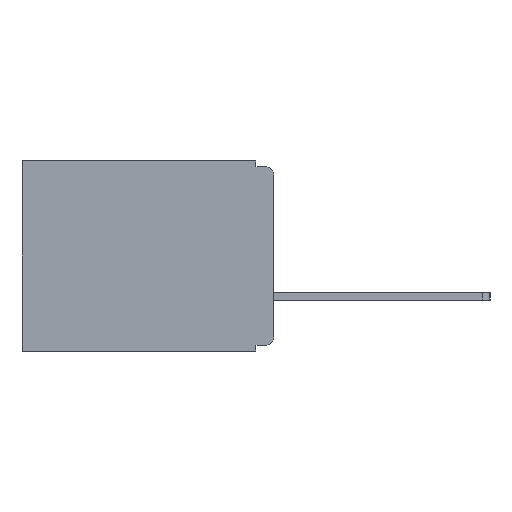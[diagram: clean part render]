
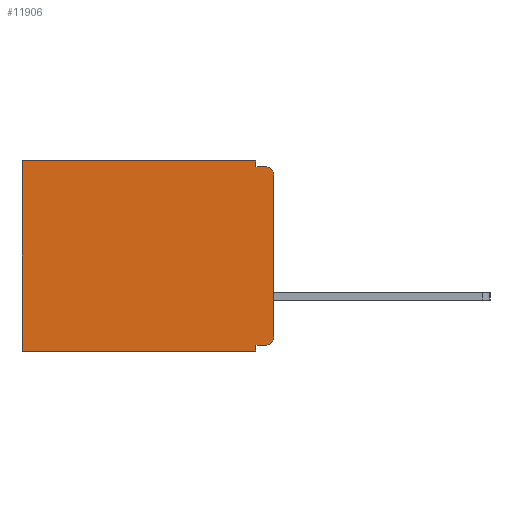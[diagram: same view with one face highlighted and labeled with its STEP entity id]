
A CAD part, left-side view. The second image highlights one B-rep face of the part: STEP entity #11906.
In plain terms, the highlighted planar face has unit normal (-1, 0, 0).
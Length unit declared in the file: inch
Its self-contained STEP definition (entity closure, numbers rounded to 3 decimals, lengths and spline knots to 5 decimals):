
#250 = AXIS2_PLACEMENT_3D ( 'NONE', #4049, #21168, #6512 ) ;
#1176 = CARTESIAN_POINT ( 'NONE',  ( 0.3, 0., -0.33 ) ) ;
#1823 = VECTOR ( 'NONE', #9104, 39.37008 ) ;
#1893 = VERTEX_POINT ( 'NONE', #15947 ) ;
#1997 = VERTEX_POINT ( 'NONE', #14978 ) ;
#2193 = EDGE_CURVE ( 'NONE', #8790, #23885, #7964, .T. ) ;
#3011 = VECTOR ( 'NONE', #12356, 39.37008 ) ;
#3123 = ORIENTED_EDGE ( 'NONE', *, *, #17317, .T. ) ;
#3446 = CARTESIAN_POINT ( 'NONE',  ( 0.3, 0.437, -0.33 ) ) ;
#3621 = ORIENTED_EDGE ( 'NONE', *, *, #25873, .T. ) ;
#4049 = CARTESIAN_POINT ( 'NONE',  ( 0.3, 0.015, -0.025 ) ) ;
#4322 = CARTESIAN_POINT ( 'NONE',  ( 0.3, 0.031, 0. ) ) ;
#4639 = CARTESIAN_POINT ( 'NONE',  ( 0.3, 0., -0.305 ) ) ;
#4737 = EDGE_LOOP ( 'NONE', ( #25357, #3621, #29561, #24576, #3123, #17322, #12227, #15535, #8916, #21653 ) ) ;
#5652 = DIRECTION ( 'NONE',  ( 0., 1., 0. ) ) ;
#6342 = DIRECTION ( 'NONE',  ( 0., 0., -1. ) ) ;
#6512 = DIRECTION ( 'NONE',  ( 0., 0., -1. ) ) ;
#6566 = CARTESIAN_POINT ( 'NONE',  ( 0.3, 0.437, -0.33 ) ) ;
#6647 = PLANE ( 'NONE',  #27971 ) ;
#7565 = EDGE_CURVE ( 'NONE', #8790, #13535, #9932, .T. ) ;
#7601 = VECTOR ( 'NONE', #6342, 39.37008 ) ;
#7878 = CARTESIAN_POINT ( 'NONE',  ( 0.3, 0.031, 0. ) ) ;
#7964 = LINE ( 'NONE', #12493, #3011 ) ;
#8508 = EDGE_CURVE ( 'NONE', #24774, #22736, #16221, .T. ) ;
#8790 = VERTEX_POINT ( 'NONE', #21721 ) ;
#8916 = ORIENTED_EDGE ( 'NONE', *, *, #2193, .F. ) ;
#9104 = DIRECTION ( 'NONE',  ( 0., 0., -1. ) ) ;
#9932 = CIRCLE ( 'NONE', #15893, 0.015 ) ;
#10618 = DIRECTION ( 'NONE',  ( 0., -1., 0. ) ) ;
#11228 = VECTOR ( 'NONE', #18077, 39.37008 ) ;
#11843 = VECTOR ( 'NONE', #5652, 39.37008 ) ;
#11906 = ADVANCED_FACE ( 'NONE', ( #29597 ), #6647, .F. ) ;
#12227 = ORIENTED_EDGE ( 'NONE', *, *, #23115, .F. ) ;
#12356 = DIRECTION ( 'NONE',  ( 0., 1., 0. ) ) ;
#12384 = EDGE_CURVE ( 'NONE', #22079, #13535, #15184, .T. ) ;
#12493 = CARTESIAN_POINT ( 'NONE',  ( 0.3, 0., -0.32 ) ) ;
#13535 = VERTEX_POINT ( 'NONE', #4639 ) ;
#13689 = CARTESIAN_POINT ( 'NONE',  ( 0.3, 0.437, 0. ) ) ;
#13719 = CARTESIAN_POINT ( 'NONE',  ( 0.3, 0., -0.025 ) ) ;
#13982 = DIRECTION ( 'NONE',  ( 1., 0., 0. ) ) ;
#14138 = LINE ( 'NONE', #25143, #11843 ) ;
#14469 = DIRECTION ( 'NONE',  ( -1., 0., 0. ) ) ;
#14978 = CARTESIAN_POINT ( 'NONE',  ( 0.3, 0.015, -0.01 ) ) ;
#15184 = LINE ( 'NONE', #1176, #28088 ) ;
#15535 = ORIENTED_EDGE ( 'NONE', *, *, #18160, .F. ) ;
#15583 = LINE ( 'NONE', #4322, #1823 ) ;
#15893 = AXIS2_PLACEMENT_3D ( 'NONE', #29004, #14469, #31358 ) ;
#15947 = CARTESIAN_POINT ( 'NONE',  ( 0.3, 0.031, -0.01 ) ) ;
#15984 = CIRCLE ( 'NONE', #250, 0.015 ) ;
#16221 = LINE ( 'NONE', #3446, #11228 ) ;
#16236 = VERTEX_POINT ( 'NONE', #23511 ) ;
#17317 = EDGE_CURVE ( 'NONE', #27216, #24774, #14138, .T. ) ;
#17322 = ORIENTED_EDGE ( 'NONE', *, *, #8508, .T. ) ;
#17855 = CARTESIAN_POINT ( 'NONE',  ( 0.3, 0., -0.33 ) ) ;
#18077 = DIRECTION ( 'NONE',  ( 0., 0., -1. ) ) ;
#18160 = EDGE_CURVE ( 'NONE', #23885, #16236, #21404, .T. ) ;
#18237 = VECTOR ( 'NONE', #10618, 39.37008 ) ;
#18266 = DIRECTION ( 'NONE',  ( 0., 0., -1. ) ) ;
#18551 = CARTESIAN_POINT ( 'NONE',  ( 0.3, 0.031, -0.32 ) ) ;
#20788 = EDGE_CURVE ( 'NONE', #27216, #1893, #15583, .T. ) ;
#21168 = DIRECTION ( 'NONE',  ( -1., 0., 0. ) ) ;
#21404 = LINE ( 'NONE', #23408, #7601 ) ;
#21577 = LINE ( 'NONE', #17855, #27195 ) ;
#21653 = ORIENTED_EDGE ( 'NONE', *, *, #7565, .T. ) ;
#21721 = CARTESIAN_POINT ( 'NONE',  ( 0.3, 0.015, -0.32 ) ) ;
#22079 = VERTEX_POINT ( 'NONE', #13719 ) ;
#22736 = VERTEX_POINT ( 'NONE', #6566 ) ;
#23115 = EDGE_CURVE ( 'NONE', #16236, #22736, #21577, .T. ) ;
#23408 = CARTESIAN_POINT ( 'NONE',  ( 0.3, 0.031, -0.33 ) ) ;
#23511 = CARTESIAN_POINT ( 'NONE',  ( 0.3, 0.031, -0.33 ) ) ;
#23885 = VERTEX_POINT ( 'NONE', #18551 ) ;
#24576 = ORIENTED_EDGE ( 'NONE', *, *, #20788, .F. ) ;
#24774 = VERTEX_POINT ( 'NONE', #13689 ) ;
#25075 = DIRECTION ( 'NONE',  ( 0., 1., 0. ) ) ;
#25143 = CARTESIAN_POINT ( 'NONE',  ( 0.3, 0., 0. ) ) ;
#25352 = CARTESIAN_POINT ( 'NONE',  ( 0.3, 0., -0.01 ) ) ;
#25357 = ORIENTED_EDGE ( 'NONE', *, *, #12384, .F. ) ;
#25456 = LINE ( 'NONE', #25352, #18237 ) ;
#25873 = EDGE_CURVE ( 'NONE', #22079, #1997, #15984, .T. ) ;
#27195 = VECTOR ( 'NONE', #25075, 39.37008 ) ;
#27216 = VERTEX_POINT ( 'NONE', #7878 ) ;
#27971 = AXIS2_PLACEMENT_3D ( 'NONE', #28539, #13982, #30896 ) ;
#28088 = VECTOR ( 'NONE', #18266, 39.37008 ) ;
#28539 = CARTESIAN_POINT ( 'NONE',  ( 0.3, 0., -0.33 ) ) ;
#29004 = CARTESIAN_POINT ( 'NONE',  ( 0.3, 0.015, -0.305 ) ) ;
#29561 = ORIENTED_EDGE ( 'NONE', *, *, #30688, .F. ) ;
#29597 = FACE_OUTER_BOUND ( 'NONE', #4737, .T. ) ;
#30688 = EDGE_CURVE ( 'NONE', #1893, #1997, #25456, .T. ) ;
#30896 = DIRECTION ( 'NONE',  ( 0., 0., -1. ) ) ;
#31358 = DIRECTION ( 'NONE',  ( 0., 0., -1. ) ) ;
